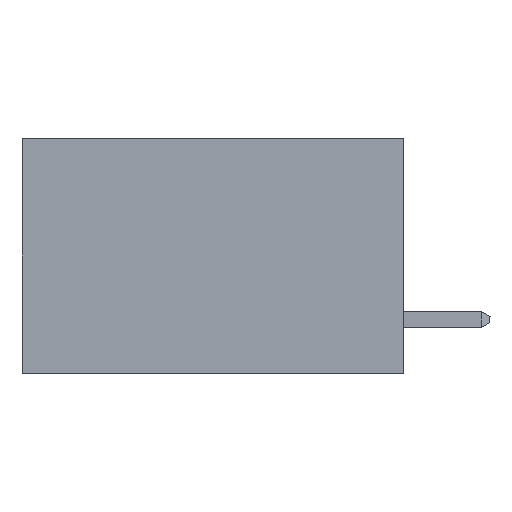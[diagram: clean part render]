
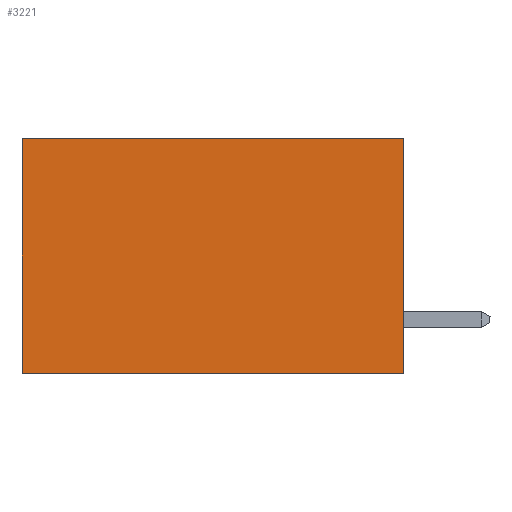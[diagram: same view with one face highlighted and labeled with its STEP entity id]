
A CAD part, left-side view. The second image highlights one B-rep face of the part: STEP entity #3221.
In plain terms, the highlighted planar face has unit normal (-1, 0, 0).
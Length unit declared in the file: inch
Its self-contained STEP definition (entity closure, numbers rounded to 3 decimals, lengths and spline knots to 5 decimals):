
#3221 = ADVANCED_FACE ( 'NONE', ( #24424 ), #23565, .F. ) ;
#5390 = ORIENTED_EDGE ( 'NONE', *, *, #14413, .T. ) ;
#8825 = DIRECTION ( 'NONE',  ( 0., 0., -1. ) ) ;
#9333 = LINE ( 'NONE', #39941, #38214 ) ;
#10623 = LINE ( 'NONE', #36318, #40630 ) ;
#11209 = EDGE_LOOP ( 'NONE', ( #5390, #25328, #41223, #16690 ) ) ;
#11827 = LINE ( 'NONE', #12943, #28789 ) ;
#12266 = VERTEX_POINT ( 'NONE', #34491 ) ;
#12943 = CARTESIAN_POINT ( 'NONE',  ( 0.2875, 0., 0. ) ) ;
#13925 = EDGE_CURVE ( 'NONE', #34199, #41713, #11827, .T. ) ;
#14413 = EDGE_CURVE ( 'NONE', #41713, #18737, #10623, .T. ) ;
#15792 = CARTESIAN_POINT ( 'NONE',  ( 0.2875, 0., 0. ) ) ;
#16690 = ORIENTED_EDGE ( 'NONE', *, *, #13925, .T. ) ;
#18737 = VERTEX_POINT ( 'NONE', #42859 ) ;
#23565 = PLANE ( 'NONE',  #38514 ) ;
#24398 = CARTESIAN_POINT ( 'NONE',  ( 0.2875, 0.6, 0. ) ) ;
#24424 = FACE_OUTER_BOUND ( 'NONE', #11209, .T. ) ;
#25328 = ORIENTED_EDGE ( 'NONE', *, *, #37921, .F. ) ;
#25726 = DIRECTION ( 'NONE',  ( 0., 0., -1. ) ) ;
#25918 = CARTESIAN_POINT ( 'NONE',  ( 0.2875, 0., -0.37 ) ) ;
#27190 = DIRECTION ( 'NONE',  ( 1., 0., 0. ) ) ;
#28789 = VECTOR ( 'NONE', #30869, 39.37008 ) ;
#29194 = DIRECTION ( 'NONE',  ( 0., 0., -1. ) ) ;
#30869 = DIRECTION ( 'NONE',  ( 0., 1., 0. ) ) ;
#34199 = VERTEX_POINT ( 'NONE', #39936 ) ;
#34491 = CARTESIAN_POINT ( 'NONE',  ( 0.2875, 0., -0.37 ) ) ;
#35096 = EDGE_CURVE ( 'NONE', #34199, #12266, #9333, .T. ) ;
#35115 = VECTOR ( 'NONE', #36648, 39.37008 ) ;
#36318 = CARTESIAN_POINT ( 'NONE',  ( 0.2875, 0.6, 0. ) ) ;
#36648 = DIRECTION ( 'NONE',  ( 0., 1., 0. ) ) ;
#37921 = EDGE_CURVE ( 'NONE', #12266, #18737, #39078, .T. ) ;
#38214 = VECTOR ( 'NONE', #29194, 39.37008 ) ;
#38514 = AXIS2_PLACEMENT_3D ( 'NONE', #15792, #27190, #8825 ) ;
#39078 = LINE ( 'NONE', #25918, #35115 ) ;
#39936 = CARTESIAN_POINT ( 'NONE',  ( 0.2875, 0., 0. ) ) ;
#39941 = CARTESIAN_POINT ( 'NONE',  ( 0.2875, 0., 0. ) ) ;
#40630 = VECTOR ( 'NONE', #25726, 39.37008 ) ;
#41223 = ORIENTED_EDGE ( 'NONE', *, *, #35096, .F. ) ;
#41713 = VERTEX_POINT ( 'NONE', #24398 ) ;
#42859 = CARTESIAN_POINT ( 'NONE',  ( 0.2875, 0.6, -0.37 ) ) ;
